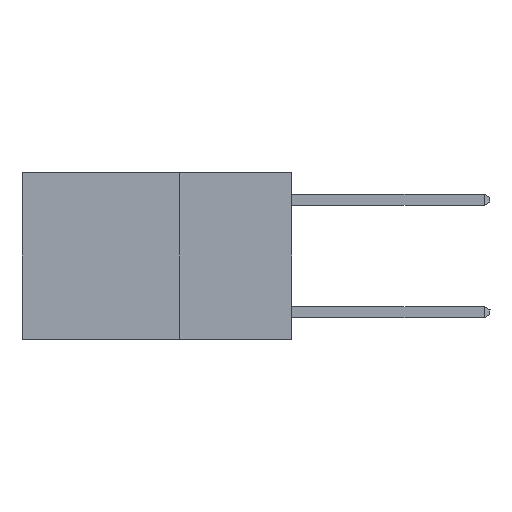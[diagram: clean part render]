
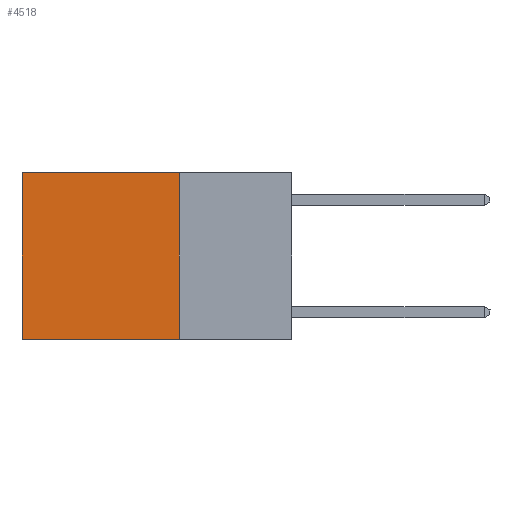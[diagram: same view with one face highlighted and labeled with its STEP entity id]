
A CAD part, left-side view. The second image highlights one B-rep face of the part: STEP entity #4518.
In plain terms, the highlighted planar face has unit normal (-1, 0, 0).
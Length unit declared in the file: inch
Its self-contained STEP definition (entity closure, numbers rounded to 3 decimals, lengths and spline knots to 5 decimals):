
#29 = VECTOR ( 'NONE', #4846, 39.37008 ) ;
#164 = FACE_OUTER_BOUND ( 'NONE', #4443, .T. ) ;
#904 = LINE ( 'NONE', #6804, #6572 ) ;
#2261 = EDGE_CURVE ( 'NONE', #7086, #5663, #904, .T. ) ;
#3423 = VECTOR ( 'NONE', #3765, 39.37008 ) ;
#3702 = LINE ( 'NONE', #9156, #29 ) ;
#3765 = DIRECTION ( 'NONE',  ( 0., 1., 0. ) ) ;
#4443 = EDGE_LOOP ( 'NONE', ( #7157, #9904, #7470, #10224 ) ) ;
#4518 = ADVANCED_FACE ( 'NONE', ( #164 ), #10729, .F. ) ;
#4846 = DIRECTION ( 'NONE',  ( 0., 0., -1. ) ) ;
#5153 = EDGE_CURVE ( 'NONE', #5663, #13430, #6178, .T. ) ;
#5476 = DIRECTION ( 'NONE',  ( 0., 0., -1. ) ) ;
#5513 = EDGE_CURVE ( 'NONE', #7086, #12426, #8960, .T. ) ;
#5663 = VERTEX_POINT ( 'NONE', #12474 ) ;
#5795 = VECTOR ( 'NONE', #12074, 39.37008 ) ;
#6178 = LINE ( 'NONE', #10270, #3423 ) ;
#6572 = VECTOR ( 'NONE', #7865, 39.37008 ) ;
#6804 = CARTESIAN_POINT ( 'NONE',  ( 0.2625, 0.25, 0. ) ) ;
#6939 = CARTESIAN_POINT ( 'NONE',  ( 0.2625, 0.25, 0. ) ) ;
#7086 = VERTEX_POINT ( 'NONE', #7397 ) ;
#7157 = ORIENTED_EDGE ( 'NONE', *, *, #9314, .T. ) ;
#7397 = CARTESIAN_POINT ( 'NONE',  ( 0.2625, 0.25, 0. ) ) ;
#7470 = ORIENTED_EDGE ( 'NONE', *, *, #2261, .F. ) ;
#7604 = CARTESIAN_POINT ( 'NONE',  ( 0.2625, 0.6, -0.37 ) ) ;
#7865 = DIRECTION ( 'NONE',  ( 0., 0., -1. ) ) ;
#8960 = LINE ( 'NONE', #6939, #5795 ) ;
#9156 = CARTESIAN_POINT ( 'NONE',  ( 0.2625, 0.6, 0. ) ) ;
#9314 = EDGE_CURVE ( 'NONE', #12426, #13430, #3702, .T. ) ;
#9693 = CARTESIAN_POINT ( 'NONE',  ( 0.2625, 0.25, 0. ) ) ;
#9904 = ORIENTED_EDGE ( 'NONE', *, *, #5153, .F. ) ;
#10224 = ORIENTED_EDGE ( 'NONE', *, *, #5513, .T. ) ;
#10270 = CARTESIAN_POINT ( 'NONE',  ( 0.2625, 0.25, -0.37 ) ) ;
#10729 = PLANE ( 'NONE',  #13019 ) ;
#11742 = DIRECTION ( 'NONE',  ( 1., 0., 0. ) ) ;
#12074 = DIRECTION ( 'NONE',  ( 0., 1., 0. ) ) ;
#12426 = VERTEX_POINT ( 'NONE', #13296 ) ;
#12474 = CARTESIAN_POINT ( 'NONE',  ( 0.2625, 0.25, -0.37 ) ) ;
#13019 = AXIS2_PLACEMENT_3D ( 'NONE', #9693, #11742, #5476 ) ;
#13296 = CARTESIAN_POINT ( 'NONE',  ( 0.2625, 0.6, 0. ) ) ;
#13430 = VERTEX_POINT ( 'NONE', #7604 ) ;
